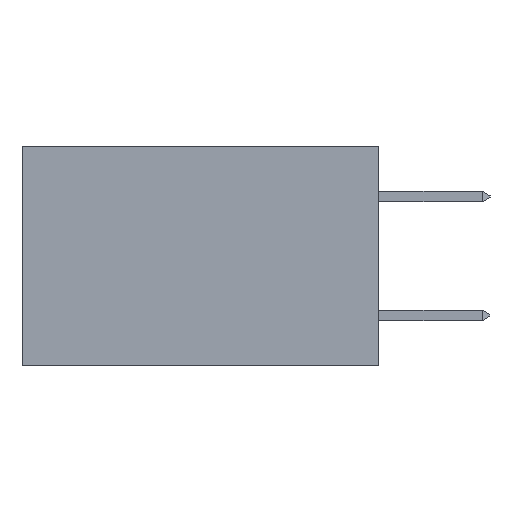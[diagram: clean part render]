
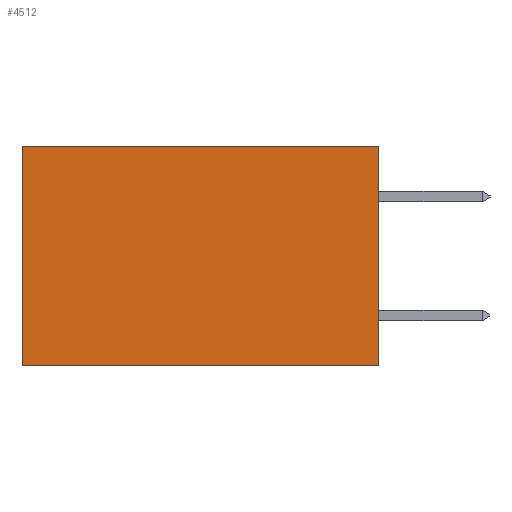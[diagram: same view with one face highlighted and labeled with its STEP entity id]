
A CAD part, left-side view. The second image highlights one B-rep face of the part: STEP entity #4512.
In plain terms, the highlighted planar face has unit normal (-1, 0, 0).
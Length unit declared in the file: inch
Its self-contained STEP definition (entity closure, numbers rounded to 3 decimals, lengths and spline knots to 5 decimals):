
#66 = CARTESIAN_POINT ( 'NONE',  ( 0.298, 0., 0. ) ) ;
#307 = DIRECTION ( 'NONE',  ( 0., 0., -1. ) ) ;
#394 = PLANE ( 'NONE',  #1516 ) ;
#613 = EDGE_CURVE ( 'NONE', #1217, #5644, #3892, .T. ) ;
#673 = VERTEX_POINT ( 'NONE', #7011 ) ;
#918 = EDGE_CURVE ( 'NONE', #1217, #673, #5824, .T. ) ;
#1217 = VERTEX_POINT ( 'NONE', #7073 ) ;
#1221 = DIRECTION ( 'NONE',  ( 0., 0., -1. ) ) ;
#1516 = AXIS2_PLACEMENT_3D ( 'NONE', #66, #1540, #307 ) ;
#1540 = DIRECTION ( 'NONE',  ( 1., 0., 0. ) ) ;
#1710 = CARTESIAN_POINT ( 'NONE',  ( 0.298, 0., 0. ) ) ;
#2381 = DIRECTION ( 'NONE',  ( 0., 1., 0. ) ) ;
#2720 = DIRECTION ( 'NONE',  ( 0., 0., -1. ) ) ;
#2738 = VECTOR ( 'NONE', #8718, 39.37008 ) ;
#2834 = ORIENTED_EDGE ( 'NONE', *, *, #10837, .F. ) ;
#3525 = ORIENTED_EDGE ( 'NONE', *, *, #918, .T. ) ;
#3626 = LINE ( 'NONE', #9486, #8706 ) ;
#3892 = LINE ( 'NONE', #1710, #8948 ) ;
#4295 = VECTOR ( 'NONE', #2720, 39.37008 ) ;
#4296 = VERTEX_POINT ( 'NONE', #9152 ) ;
#4512 = ADVANCED_FACE ( 'NONE', ( #11902 ), #394, .F. ) ;
#4961 = LINE ( 'NONE', #6882, #4295 ) ;
#5058 = ORIENTED_EDGE ( 'NONE', *, *, #9856, .T. ) ;
#5644 = VERTEX_POINT ( 'NONE', #6150 ) ;
#5768 = CARTESIAN_POINT ( 'NONE',  ( 0.298, 0., 0. ) ) ;
#5824 = LINE ( 'NONE', #5768, #2738 ) ;
#5931 = EDGE_LOOP ( 'NONE', ( #5058, #2834, #10357, #3525 ) ) ;
#6150 = CARTESIAN_POINT ( 'NONE',  ( 0.298, 0., -0.37 ) ) ;
#6882 = CARTESIAN_POINT ( 'NONE',  ( 0.298, 0.6, 0. ) ) ;
#7011 = CARTESIAN_POINT ( 'NONE',  ( 0.298, 0.6, 0. ) ) ;
#7073 = CARTESIAN_POINT ( 'NONE',  ( 0.298, 0., 0. ) ) ;
#8706 = VECTOR ( 'NONE', #2381, 39.37008 ) ;
#8718 = DIRECTION ( 'NONE',  ( 0., 1., 0. ) ) ;
#8948 = VECTOR ( 'NONE', #1221, 39.37008 ) ;
#9152 = CARTESIAN_POINT ( 'NONE',  ( 0.298, 0.6, -0.37 ) ) ;
#9486 = CARTESIAN_POINT ( 'NONE',  ( 0.298, 0., -0.37 ) ) ;
#9856 = EDGE_CURVE ( 'NONE', #673, #4296, #4961, .T. ) ;
#10357 = ORIENTED_EDGE ( 'NONE', *, *, #613, .F. ) ;
#10837 = EDGE_CURVE ( 'NONE', #5644, #4296, #3626, .T. ) ;
#11902 = FACE_OUTER_BOUND ( 'NONE', #5931, .T. ) ;
